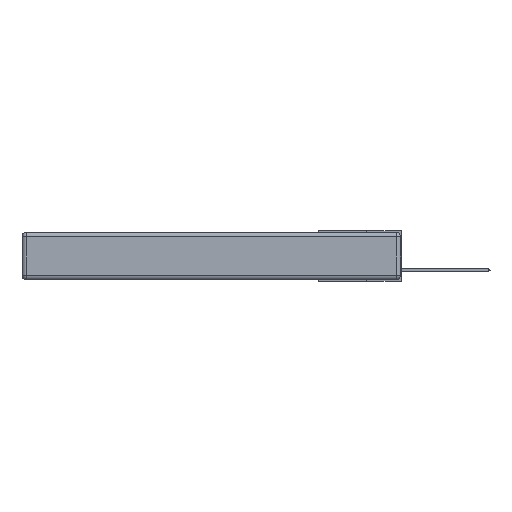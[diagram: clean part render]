
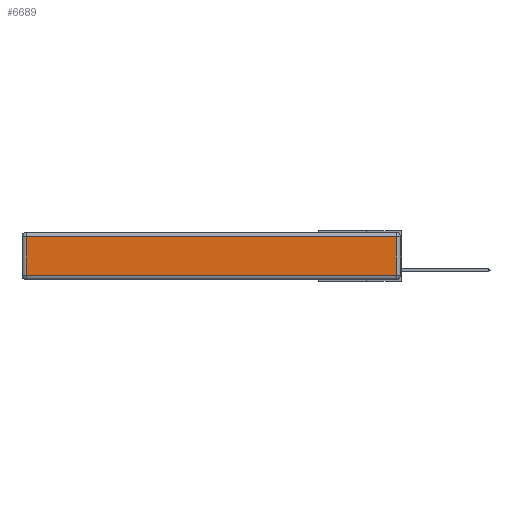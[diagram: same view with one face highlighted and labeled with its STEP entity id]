
A CAD part, left-side view. The second image highlights one B-rep face of the part: STEP entity #6689.
In plain terms, the highlighted planar face has unit normal (-1, 0, 0).
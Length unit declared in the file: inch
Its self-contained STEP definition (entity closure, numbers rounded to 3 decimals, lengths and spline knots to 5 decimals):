
#208 = EDGE_CURVE ( 'NONE', #7875, #2065, #7362, .T. ) ;
#776 = LINE ( 'NONE', #8921, #6876 ) ;
#1181 = ORIENTED_EDGE ( 'NONE', *, *, #12901, .T. ) ;
#1316 = DIRECTION ( 'NONE',  ( -1., 0., 0. ) ) ;
#1523 = LINE ( 'NONE', #9254, #13239 ) ;
#2065 = VERTEX_POINT ( 'NONE', #2526 ) ;
#2371 = EDGE_LOOP ( 'NONE', ( #13795, #1181, #8598, #6842 ) ) ;
#2526 = CARTESIAN_POINT ( 'NONE',  ( 0., 0.03, -0.313 ) ) ;
#2741 = VERTEX_POINT ( 'NONE', #14523 ) ;
#2844 = CARTESIAN_POINT ( 'NONE',  ( 0., 0., -0.343 ) ) ;
#3378 = CARTESIAN_POINT ( 'NONE',  ( 0., 0., -0.313 ) ) ;
#3546 = CARTESIAN_POINT ( 'NONE',  ( 0., 2.72, -0.313 ) ) ;
#3727 = VERTEX_POINT ( 'NONE', #11820 ) ;
#4315 = EDGE_CURVE ( 'NONE', #3727, #2741, #776, .T. ) ;
#6689 = ADVANCED_FACE ( 'NONE', ( #11140 ), #17793, .T. ) ;
#6842 = ORIENTED_EDGE ( 'NONE', *, *, #17327, .T. ) ;
#6876 = VECTOR ( 'NONE', #10384, 39.37008 ) ;
#6902 = VECTOR ( 'NONE', #13244, 39.37008 ) ;
#7362 = LINE ( 'NONE', #3378, #16054 ) ;
#7875 = VERTEX_POINT ( 'NONE', #3546 ) ;
#8598 = ORIENTED_EDGE ( 'NONE', *, *, #4315, .T. ) ;
#8921 = CARTESIAN_POINT ( 'NONE',  ( 0., 2.75, -0.03 ) ) ;
#9254 = CARTESIAN_POINT ( 'NONE',  ( 0., 0.03, -0.343 ) ) ;
#10384 = DIRECTION ( 'NONE',  ( 0., 1., 0. ) ) ;
#11140 = FACE_OUTER_BOUND ( 'NONE', #2371, .T. ) ;
#11820 = CARTESIAN_POINT ( 'NONE',  ( 0., 0.03, -0.03 ) ) ;
#12901 = EDGE_CURVE ( 'NONE', #2065, #3727, #1523, .T. ) ;
#12906 = AXIS2_PLACEMENT_3D ( 'NONE', #2844, #1316, #13906 ) ;
#13239 = VECTOR ( 'NONE', #16413, 39.37008 ) ;
#13244 = DIRECTION ( 'NONE',  ( 0., 0., -1. ) ) ;
#13795 = ORIENTED_EDGE ( 'NONE', *, *, #208, .T. ) ;
#13906 = DIRECTION ( 'NONE',  ( 0., 0., 1. ) ) ;
#14523 = CARTESIAN_POINT ( 'NONE',  ( 0., 2.72, -0.03 ) ) ;
#14545 = DIRECTION ( 'NONE',  ( 0., -1., 0. ) ) ;
#16028 = LINE ( 'NONE', #16101, #6902 ) ;
#16054 = VECTOR ( 'NONE', #14545, 39.37008 ) ;
#16101 = CARTESIAN_POINT ( 'NONE',  ( 0., 2.72, -0.343 ) ) ;
#16413 = DIRECTION ( 'NONE',  ( 0., 0., 1. ) ) ;
#17327 = EDGE_CURVE ( 'NONE', #2741, #7875, #16028, .T. ) ;
#17793 = PLANE ( 'NONE',  #12906 ) ;
